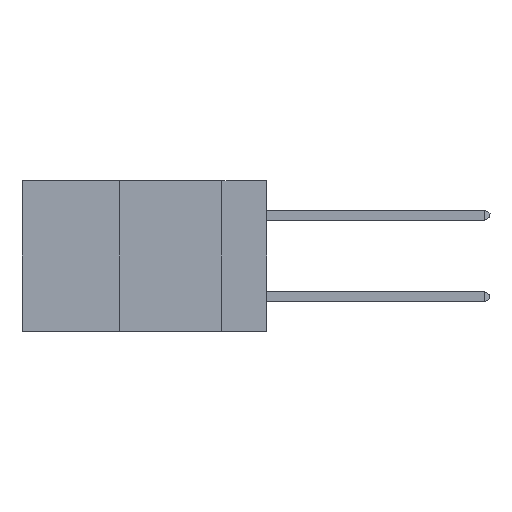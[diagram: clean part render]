
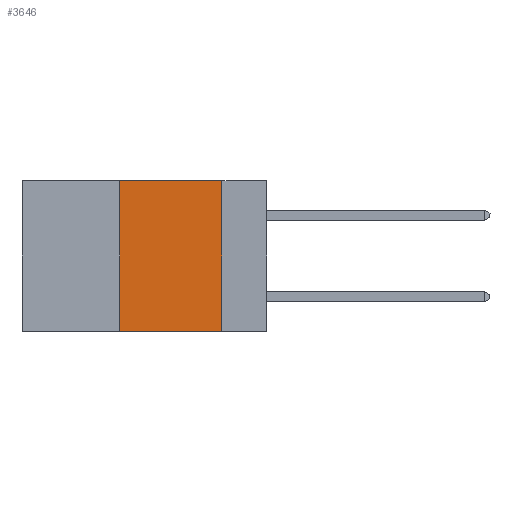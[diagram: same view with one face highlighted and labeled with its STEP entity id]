
A CAD part, left-side view. The second image highlights one B-rep face of the part: STEP entity #3646.
In plain terms, the highlighted planar face has unit normal (-1, 0, 0).
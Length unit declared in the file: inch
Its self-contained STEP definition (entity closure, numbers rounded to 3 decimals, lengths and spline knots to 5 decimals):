
#544 = ORIENTED_EDGE ( 'NONE', *, *, #7973, .T. ) ;
#857 = EDGE_CURVE ( 'NONE', #7592, #2715, #7805, .T. ) ;
#1187 = ORIENTED_EDGE ( 'NONE', *, *, #857, .F. ) ;
#1599 = ORIENTED_EDGE ( 'NONE', *, *, #7724, .F. ) ;
#2204 = VECTOR ( 'NONE', #10183, 39.37008 ) ;
#2473 = DIRECTION ( 'NONE',  ( 0., 0., -1. ) ) ;
#2556 = CARTESIAN_POINT ( 'NONE',  ( 0., 0.6, -0.37 ) ) ;
#2598 = DIRECTION ( 'NONE',  ( 1., 0., 0. ) ) ;
#2611 = CARTESIAN_POINT ( 'NONE',  ( 0., 0.6, 0. ) ) ;
#2682 = PLANE ( 'NONE',  #2723 ) ;
#2715 = VERTEX_POINT ( 'NONE', #6538 ) ;
#2723 = AXIS2_PLACEMENT_3D ( 'NONE', #2611, #2598, #2473 ) ;
#3321 = CARTESIAN_POINT ( 'NONE',  ( 0., 0.36, 0. ) ) ;
#3540 = VERTEX_POINT ( 'NONE', #8566 ) ;
#3646 = ADVANCED_FACE ( 'NONE', ( #8907 ), #2682, .F. ) ;
#3689 = VECTOR ( 'NONE', #4972, 39.37008 ) ;
#4456 = VECTOR ( 'NONE', #8131, 39.37008 ) ;
#4727 = LINE ( 'NONE', #6664, #2204 ) ;
#4972 = DIRECTION ( 'NONE',  ( 0., -1., 0. ) ) ;
#6422 = EDGE_LOOP ( 'NONE', ( #1599, #1187, #7631, #544 ) ) ;
#6538 = CARTESIAN_POINT ( 'NONE',  ( 0., 0.11, 0. ) ) ;
#6664 = CARTESIAN_POINT ( 'NONE',  ( 0., 0.11, 0. ) ) ;
#7592 = VERTEX_POINT ( 'NONE', #3321 ) ;
#7631 = ORIENTED_EDGE ( 'NONE', *, *, #7741, .F. ) ;
#7724 = EDGE_CURVE ( 'NONE', #2715, #8890, #4727, .T. ) ;
#7741 = EDGE_CURVE ( 'NONE', #3540, #7592, #8341, .T. ) ;
#7805 = LINE ( 'NONE', #8019, #3689 ) ;
#7973 = EDGE_CURVE ( 'NONE', #3540, #8890, #10375, .T. ) ;
#8019 = CARTESIAN_POINT ( 'NONE',  ( 0., 0.6, 0. ) ) ;
#8120 = VECTOR ( 'NONE', #9565, 39.37008 ) ;
#8131 = DIRECTION ( 'NONE',  ( 0., 0., 1. ) ) ;
#8341 = LINE ( 'NONE', #8859, #4456 ) ;
#8566 = CARTESIAN_POINT ( 'NONE',  ( 0., 0.36, -0.37 ) ) ;
#8859 = CARTESIAN_POINT ( 'NONE',  ( 0., 0.36, 0. ) ) ;
#8890 = VERTEX_POINT ( 'NONE', #9784 ) ;
#8907 = FACE_OUTER_BOUND ( 'NONE', #6422, .T. ) ;
#9565 = DIRECTION ( 'NONE',  ( 0., -1., 0. ) ) ;
#9784 = CARTESIAN_POINT ( 'NONE',  ( 0., 0.11, -0.37 ) ) ;
#10183 = DIRECTION ( 'NONE',  ( 0., 0., -1. ) ) ;
#10375 = LINE ( 'NONE', #2556, #8120 ) ;
